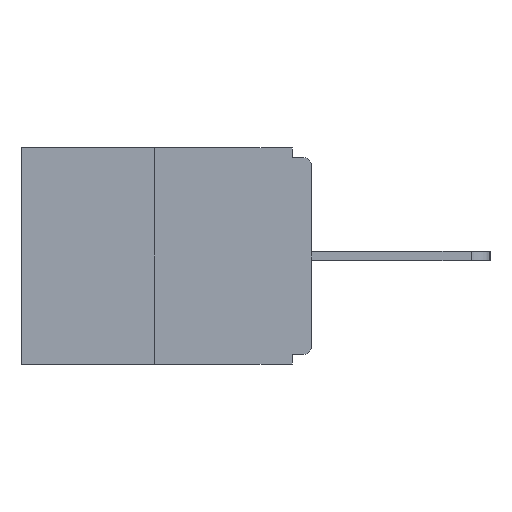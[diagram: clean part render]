
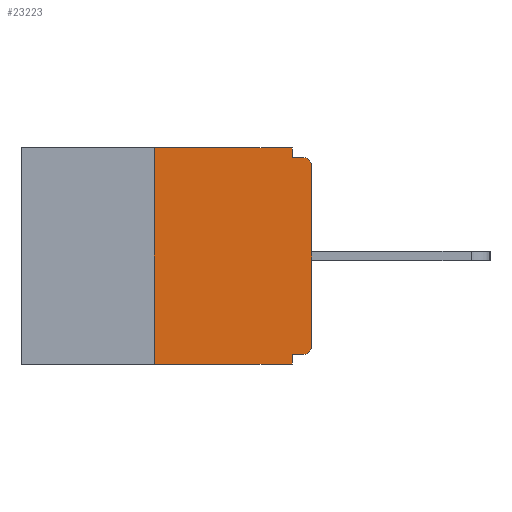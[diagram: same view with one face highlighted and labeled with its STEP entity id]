
A CAD part, left-side view. The second image highlights one B-rep face of the part: STEP entity #23223.
In plain terms, the highlighted planar face has unit normal (-1, 0, 0).
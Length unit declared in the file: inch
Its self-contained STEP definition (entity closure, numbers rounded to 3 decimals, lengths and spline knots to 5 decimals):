
#381 = CARTESIAN_POINT ( 'NONE',  ( 0., 0.25, 0. ) ) ;
#409 = DIRECTION ( 'NONE',  ( 0., 0., -1. ) ) ;
#1017 = LINE ( 'NONE', #16493, #21958 ) ;
#1474 = ORIENTED_EDGE ( 'NONE', *, *, #22453, .F. ) ;
#1804 = VECTOR ( 'NONE', #11525, 39.37008 ) ;
#1848 = CARTESIAN_POINT ( 'NONE',  ( 0., 0., -0.328 ) ) ;
#1960 = VERTEX_POINT ( 'NONE', #4333 ) ;
#2164 = VERTEX_POINT ( 'NONE', #9880 ) ;
#2498 = CARTESIAN_POINT ( 'NONE',  ( 0., 0., -0.03 ) ) ;
#2651 = CARTESIAN_POINT ( 'NONE',  ( 0., 0., -0.313 ) ) ;
#2706 = AXIS2_PLACEMENT_3D ( 'NONE', #23360, #11837, #409 ) ;
#2878 = CIRCLE ( 'NONE', #4361, 0.015 ) ;
#2885 = VECTOR ( 'NONE', #22798, 39.37008 ) ;
#3010 = DIRECTION ( 'NONE',  ( 0., 0., 1. ) ) ;
#3512 = AXIS2_PLACEMENT_3D ( 'NONE', #16083, #15774, #21845 ) ;
#3543 = EDGE_CURVE ( 'NONE', #5068, #21273, #8918, .T. ) ;
#4018 = EDGE_CURVE ( 'NONE', #21273, #4540, #9493, .T. ) ;
#4333 = CARTESIAN_POINT ( 'NONE',  ( 0., 0.031, 0. ) ) ;
#4361 = AXIS2_PLACEMENT_3D ( 'NONE', #12429, #10344, #4783 ) ;
#4463 = ORIENTED_EDGE ( 'NONE', *, *, #20393, .T. ) ;
#4540 = VERTEX_POINT ( 'NONE', #15381 ) ;
#4783 = DIRECTION ( 'NONE',  ( 0., 0., -1. ) ) ;
#5030 = LINE ( 'NONE', #1848, #15156 ) ;
#5068 = VERTEX_POINT ( 'NONE', #2651 ) ;
#5296 = DIRECTION ( 'NONE',  ( 0., 0., -1. ) ) ;
#5450 = CARTESIAN_POINT ( 'NONE',  ( 0., 0.031, 0. ) ) ;
#5549 = CARTESIAN_POINT ( 'NONE',  ( 0., 0.25, 0. ) ) ;
#5630 = VECTOR ( 'NONE', #11256, 39.37008 ) ;
#5648 = ORIENTED_EDGE ( 'NONE', *, *, #15513, .F. ) ;
#5741 = VECTOR ( 'NONE', #5296, 39.37008 ) ;
#6551 = EDGE_CURVE ( 'NONE', #7734, #5068, #2878, .T. ) ;
#6909 = LINE ( 'NONE', #5450, #5741 ) ;
#7419 = DIRECTION ( 'NONE',  ( 0., -1., 0. ) ) ;
#7734 = VERTEX_POINT ( 'NONE', #8428 ) ;
#8182 = VERTEX_POINT ( 'NONE', #381 ) ;
#8428 = CARTESIAN_POINT ( 'NONE',  ( 0., 0.015, -0.328 ) ) ;
#8918 = LINE ( 'NONE', #20886, #23697 ) ;
#9054 = EDGE_CURVE ( 'NONE', #20295, #4540, #1017, .T. ) ;
#9493 = CIRCLE ( 'NONE', #3512, 0.015 ) ;
#9880 = CARTESIAN_POINT ( 'NONE',  ( 0., 0.25, -0.343 ) ) ;
#10344 = DIRECTION ( 'NONE',  ( -1., 0., 0. ) ) ;
#10521 = FACE_OUTER_BOUND ( 'NONE', #17765, .T. ) ;
#11256 = DIRECTION ( 'NONE',  ( 0., -1., 0. ) ) ;
#11296 = ORIENTED_EDGE ( 'NONE', *, *, #6551, .T. ) ;
#11525 = DIRECTION ( 'NONE',  ( 0., 0., -1. ) ) ;
#11837 = DIRECTION ( 'NONE',  ( 1., 0., 0. ) ) ;
#12429 = CARTESIAN_POINT ( 'NONE',  ( 0., 0.015, -0.313 ) ) ;
#12707 = LINE ( 'NONE', #15049, #22331 ) ;
#14903 = ORIENTED_EDGE ( 'NONE', *, *, #3543, .T. ) ;
#15049 = CARTESIAN_POINT ( 'NONE',  ( 0., 0.46, 0. ) ) ;
#15156 = VECTOR ( 'NONE', #15175, 39.37008 ) ;
#15175 = DIRECTION ( 'NONE',  ( 0., 1., 0. ) ) ;
#15381 = CARTESIAN_POINT ( 'NONE',  ( 0., 0.015, -0.015 ) ) ;
#15471 = VERTEX_POINT ( 'NONE', #22600 ) ;
#15513 = EDGE_CURVE ( 'NONE', #7734, #24011, #5030, .T. ) ;
#15774 = DIRECTION ( 'NONE',  ( -1., 0., 0. ) ) ;
#16083 = CARTESIAN_POINT ( 'NONE',  ( 0., 0.015, -0.03 ) ) ;
#16330 = LINE ( 'NONE', #22774, #5630 ) ;
#16493 = CARTESIAN_POINT ( 'NONE',  ( 0., 0., -0.015 ) ) ;
#16636 = ORIENTED_EDGE ( 'NONE', *, *, #21660, .F. ) ;
#16987 = LINE ( 'NONE', #19182, #1804 ) ;
#17394 = EDGE_CURVE ( 'NONE', #1960, #20295, #6909, .T. ) ;
#17765 = EDGE_LOOP ( 'NONE', ( #1474, #16636, #4463, #20351, #5648, #11296, #14903, #22760, #23952, #20081 ) ) ;
#17992 = CARTESIAN_POINT ( 'NONE',  ( 0., 0.031, -0.328 ) ) ;
#18495 = DIRECTION ( 'NONE',  ( 0., -1., 0. ) ) ;
#18723 = EDGE_CURVE ( 'NONE', #24011, #15471, #16987, .T. ) ;
#19182 = CARTESIAN_POINT ( 'NONE',  ( 0., 0.031, -0.343 ) ) ;
#20081 = ORIENTED_EDGE ( 'NONE', *, *, #17394, .F. ) ;
#20295 = VERTEX_POINT ( 'NONE', #22451 ) ;
#20351 = ORIENTED_EDGE ( 'NONE', *, *, #18723, .F. ) ;
#20393 = EDGE_CURVE ( 'NONE', #2164, #15471, #16330, .T. ) ;
#20886 = CARTESIAN_POINT ( 'NONE',  ( 0., 0., 0. ) ) ;
#21273 = VERTEX_POINT ( 'NONE', #2498 ) ;
#21430 = PLANE ( 'NONE',  #2706 ) ;
#21660 = EDGE_CURVE ( 'NONE', #2164, #8182, #23244, .T. ) ;
#21845 = DIRECTION ( 'NONE',  ( 0., 0., -1. ) ) ;
#21958 = VECTOR ( 'NONE', #18495, 39.37008 ) ;
#22331 = VECTOR ( 'NONE', #7419, 39.37008 ) ;
#22451 = CARTESIAN_POINT ( 'NONE',  ( 0., 0.031, -0.015 ) ) ;
#22453 = EDGE_CURVE ( 'NONE', #8182, #1960, #12707, .T. ) ;
#22600 = CARTESIAN_POINT ( 'NONE',  ( 0., 0.031, -0.343 ) ) ;
#22760 = ORIENTED_EDGE ( 'NONE', *, *, #4018, .T. ) ;
#22774 = CARTESIAN_POINT ( 'NONE',  ( 0., 0.46, -0.343 ) ) ;
#22798 = DIRECTION ( 'NONE',  ( 0., 0., 1. ) ) ;
#23223 = ADVANCED_FACE ( 'NONE', ( #10521 ), #21430, .F. ) ;
#23244 = LINE ( 'NONE', #5549, #2885 ) ;
#23360 = CARTESIAN_POINT ( 'NONE',  ( 0., 0.46, 0. ) ) ;
#23697 = VECTOR ( 'NONE', #3010, 39.37008 ) ;
#23952 = ORIENTED_EDGE ( 'NONE', *, *, #9054, .F. ) ;
#24011 = VERTEX_POINT ( 'NONE', #17992 ) ;
